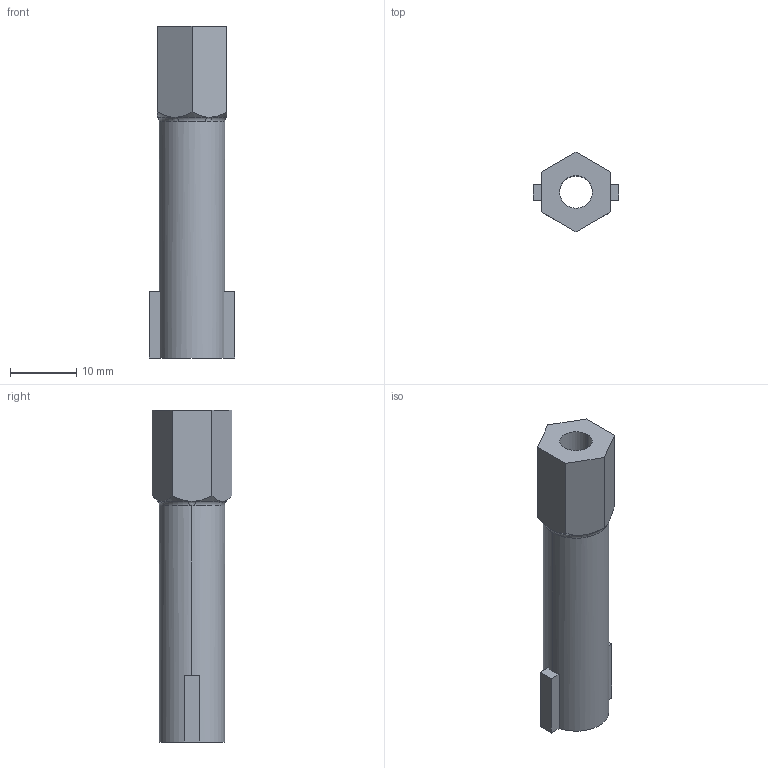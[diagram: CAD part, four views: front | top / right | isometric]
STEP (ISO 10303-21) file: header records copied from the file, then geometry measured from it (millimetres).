
FILE_DESCRIPTION (( 'STEP AP214' ), '1' );
FILE_NAME ('Barrel111^Launcher_1.STEP', '2014-10-07T00:04:24', ( 'WarFairy' ), ( '' ), 'SwSTEP 2.0', 'SolidWorks 2013', '' );
FILE_SCHEMA (( 'AUTOMOTIVE_DESIGN' ));
Length unit declared in the file: millimetre
Products named in the file (1): Barrel111^Launcher_1
Bounding box: 12.9 x 12 x 50 mm (x, y, z)
Volume: 3064.4 mm3; surface area: 2644.9 mm2
Topology: 1 solids, 1 shells, 44 faces, 108 edges, 68 vertices
Faces by surface type: plane 18, cylinder 8, cone 6, bspline 6, torus 6
Entity records: 1416 total; most frequent: CARTESIAN_POINT 377, ORIENTED_EDGE 216, DIRECTION 202, EDGE_CURVE 108, AXIS2_PLACEMENT_3D 81, VERTEX_POINT 68, EDGE_LOOP 48, ADVANCED_FACE 44
